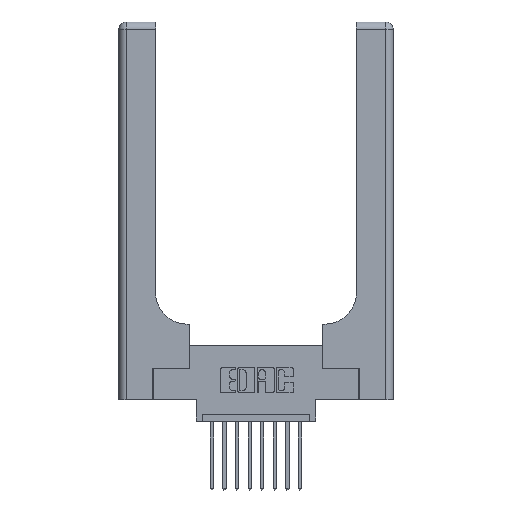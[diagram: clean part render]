
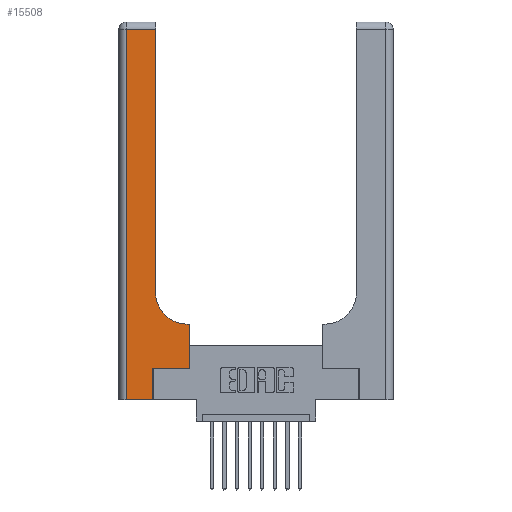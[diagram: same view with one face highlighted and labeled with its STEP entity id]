
A CAD part, top view. The second image highlights one B-rep face of the part: STEP entity #15508.
In plain terms, the highlighted planar face has unit normal (0, 0, 1).
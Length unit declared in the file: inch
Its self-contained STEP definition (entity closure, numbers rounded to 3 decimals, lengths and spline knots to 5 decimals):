
#306 = DIRECTION ( 'NONE',  ( -1., 0., 0. ) ) ;
#568 = CARTESIAN_POINT ( 'NONE',  ( 0.269, 0.25, 0.37 ) ) ;
#961 = ORIENTED_EDGE ( 'NONE', *, *, #13275, .T. ) ;
#1833 = DIRECTION ( 'NONE',  ( 0., 1., 0. ) ) ;
#1976 = LINE ( 'NONE', #6846, #11815 ) ;
#2049 = LINE ( 'NONE', #14109, #3605 ) ;
#2250 = EDGE_CURVE ( 'NONE', #15835, #10136, #14637, .T. ) ;
#2577 = DIRECTION ( 'NONE',  ( 0., 0., -1. ) ) ;
#2829 = VERTEX_POINT ( 'NONE', #8885 ) ;
#3065 = CARTESIAN_POINT ( 'NONE',  ( 0.5585, 0.25, 0.37 ) ) ;
#3093 = CARTESIAN_POINT ( 'NONE',  ( 0.5585, 0.25, 0.37 ) ) ;
#3605 = VECTOR ( 'NONE', #10420, 39.37008 ) ;
#3650 = LINE ( 'NONE', #5333, #11000 ) ;
#3883 = CARTESIAN_POINT ( 'NONE',  ( 0.2915, 0.85, 0.37 ) ) ;
#3922 = VERTEX_POINT ( 'NONE', #9143 ) ;
#4334 = CARTESIAN_POINT ( 'NONE',  ( 0.269, 0.25, 0.37 ) ) ;
#4697 = VERTEX_POINT ( 'NONE', #11025 ) ;
#4913 = CARTESIAN_POINT ( 'NONE',  ( 0., 0., 0.37 ) ) ;
#4917 = LINE ( 'NONE', #5530, #8583 ) ;
#4952 = CARTESIAN_POINT ( 'NONE',  ( 0., 3., 0.37 ) ) ;
#5185 = ORIENTED_EDGE ( 'NONE', *, *, #11216, .T. ) ;
#5333 = CARTESIAN_POINT ( 'NONE',  ( 0.06, 3., 0.37 ) ) ;
#5495 = VERTEX_POINT ( 'NONE', #6119 ) ;
#5530 = CARTESIAN_POINT ( 'NONE',  ( 0.2915, 3., 0.37 ) ) ;
#6067 = VERTEX_POINT ( 'NONE', #12944 ) ;
#6119 = CARTESIAN_POINT ( 'NONE',  ( 0.5585, 0.6, 0.37 ) ) ;
#6166 = DIRECTION ( 'NONE',  ( 0., 0., -1. ) ) ;
#6846 = CARTESIAN_POINT ( 'NONE',  ( 0., 2.94, 0.37 ) ) ;
#7076 = ORIENTED_EDGE ( 'NONE', *, *, #10704, .T. ) ;
#7225 = LINE ( 'NONE', #4334, #15515 ) ;
#7352 = CARTESIAN_POINT ( 'NONE',  ( 0.5415, 0.85, 0.37 ) ) ;
#7393 = DIRECTION ( 'NONE',  ( 1., 0., 0. ) ) ;
#7491 = VECTOR ( 'NONE', #1833, 39.37008 ) ;
#7881 = VERTEX_POINT ( 'NONE', #3065 ) ;
#8087 = DIRECTION ( 'NONE',  ( -1., 0., 0. ) ) ;
#8583 = VECTOR ( 'NONE', #11569, 39.37008 ) ;
#8695 = VERTEX_POINT ( 'NONE', #3883 ) ;
#8885 = CARTESIAN_POINT ( 'NONE',  ( 0.2915, 2.94, 0.37 ) ) ;
#9004 = ORIENTED_EDGE ( 'NONE', *, *, #12758, .T. ) ;
#9143 = CARTESIAN_POINT ( 'NONE',  ( 0.5415, 0.6, 0.37 ) ) ;
#9179 = ORIENTED_EDGE ( 'NONE', *, *, #2250, .T. ) ;
#10136 = VERTEX_POINT ( 'NONE', #568 ) ;
#10279 = CARTESIAN_POINT ( 'NONE',  ( 0.269, 0., 0.37 ) ) ;
#10420 = DIRECTION ( 'NONE',  ( -1., 0., 0. ) ) ;
#10697 = EDGE_CURVE ( 'NONE', #8695, #2829, #4917, .T. ) ;
#10704 = EDGE_CURVE ( 'NONE', #5495, #3922, #2049, .T. ) ;
#10838 = VECTOR ( 'NONE', #15509, 39.37008 ) ;
#10972 = AXIS2_PLACEMENT_3D ( 'NONE', #4952, #2577, #306 ) ;
#11000 = VECTOR ( 'NONE', #11317, 39.37008 ) ;
#11025 = CARTESIAN_POINT ( 'NONE',  ( 0.06, 0., 0.37 ) ) ;
#11216 = EDGE_CURVE ( 'NONE', #10136, #7881, #7225, .T. ) ;
#11256 = LINE ( 'NONE', #4913, #15276 ) ;
#11317 = DIRECTION ( 'NONE',  ( 0., -1., 0. ) ) ;
#11569 = DIRECTION ( 'NONE',  ( 0., 1., 0. ) ) ;
#11815 = VECTOR ( 'NONE', #8087, 39.37008 ) ;
#12414 = PLANE ( 'NONE',  #10972 ) ;
#12758 = EDGE_CURVE ( 'NONE', #4697, #15835, #11256, .T. ) ;
#12914 = LINE ( 'NONE', #3093, #7491 ) ;
#12944 = CARTESIAN_POINT ( 'NONE',  ( 0.06, 2.94, 0.37 ) ) ;
#12959 = DIRECTION ( 'NONE',  ( 1., 0., 0. ) ) ;
#13086 = CARTESIAN_POINT ( 'NONE',  ( 0.269, 0., 0.37 ) ) ;
#13275 = EDGE_CURVE ( 'NONE', #2829, #6067, #1976, .T. ) ;
#13654 = CIRCLE ( 'NONE', #14415, 0.25 ) ;
#13834 = FACE_OUTER_BOUND ( 'NONE', #14612, .T. ) ;
#13941 = ORIENTED_EDGE ( 'NONE', *, *, #14340, .T. ) ;
#14109 = CARTESIAN_POINT ( 'NONE',  ( 0.2915, 0.6, 0.37 ) ) ;
#14340 = EDGE_CURVE ( 'NONE', #7881, #5495, #12914, .T. ) ;
#14415 = AXIS2_PLACEMENT_3D ( 'NONE', #7352, #6166, #14780 ) ;
#14612 = EDGE_LOOP ( 'NONE', ( #15874, #961, #15383, #9004, #9179, #5185, #13941, #7076, #15850 ) ) ;
#14637 = LINE ( 'NONE', #13086, #10838 ) ;
#14744 = EDGE_CURVE ( 'NONE', #3922, #8695, #13654, .T. ) ;
#14780 = DIRECTION ( 'NONE',  ( 1., 0., 0. ) ) ;
#14945 = EDGE_CURVE ( 'NONE', #6067, #4697, #3650, .T. ) ;
#15276 = VECTOR ( 'NONE', #7393, 39.37008 ) ;
#15383 = ORIENTED_EDGE ( 'NONE', *, *, #14945, .T. ) ;
#15508 = ADVANCED_FACE ( 'NONE', ( #13834 ), #12414, .F. ) ;
#15509 = DIRECTION ( 'NONE',  ( 0., 1., 0. ) ) ;
#15515 = VECTOR ( 'NONE', #12959, 39.37008 ) ;
#15835 = VERTEX_POINT ( 'NONE', #10279 ) ;
#15850 = ORIENTED_EDGE ( 'NONE', *, *, #14744, .T. ) ;
#15874 = ORIENTED_EDGE ( 'NONE', *, *, #10697, .T. ) ;
